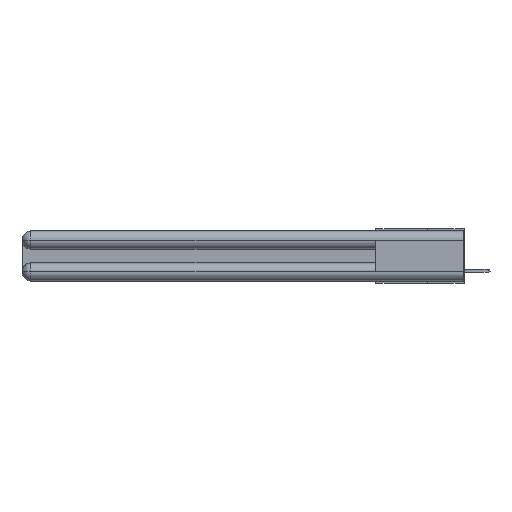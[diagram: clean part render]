
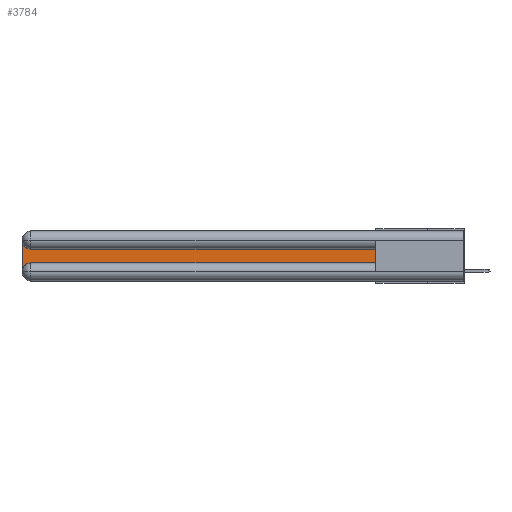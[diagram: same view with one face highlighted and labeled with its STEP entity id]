
A CAD part, left-side view. The second image highlights one B-rep face of the part: STEP entity #3784.
In plain terms, the highlighted planar face has unit normal (-1, 0, 0).
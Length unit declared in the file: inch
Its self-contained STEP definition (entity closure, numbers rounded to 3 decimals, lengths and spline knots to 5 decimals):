
#15 = DIRECTION ( 'NONE',  ( 0., 0., -1. ) ) ;
#426 = VERTEX_POINT ( 'NONE', #9883 ) ;
#629 = ORIENTED_EDGE ( 'NONE', *, *, #4254, .T. ) ;
#3064 = VECTOR ( 'NONE', #15, 39.37008 ) ;
#3088 = DIRECTION ( 'NONE',  ( 0., 0., 1. ) ) ;
#3164 = DIRECTION ( 'NONE',  ( 0., 0., -1. ) ) ;
#3468 = CARTESIAN_POINT ( 'NONE',  ( 0.075, 2.94, -0.2175 ) ) ;
#3784 = ADVANCED_FACE ( 'NONE', ( #25597 ), #5959, .F. ) ;
#4254 = EDGE_CURVE ( 'NONE', #11741, #12722, #5095, .T. ) ;
#5095 = LINE ( 'NONE', #17386, #11734 ) ;
#5959 = PLANE ( 'NONE',  #22119 ) ;
#6924 = CARTESIAN_POINT ( 'NONE',  ( 0.075, 3., -0.2175 ) ) ;
#7071 = CARTESIAN_POINT ( 'NONE',  ( 0.075, 2.94, -0.1225 ) ) ;
#8225 = EDGE_CURVE ( 'NONE', #12722, #13581, #26494, .T. ) ;
#8523 = ORIENTED_EDGE ( 'NONE', *, *, #22843, .T. ) ;
#9883 = CARTESIAN_POINT ( 'NONE',  ( 0.075, 3., -0.0625 ) ) ;
#11553 = DIRECTION ( 'NONE',  ( 0., 1., 0. ) ) ;
#11734 = VECTOR ( 'NONE', #3088, 39.37008 ) ;
#11741 = VERTEX_POINT ( 'NONE', #19174 ) ;
#12194 = VERTEX_POINT ( 'NONE', #16092 ) ;
#12722 = VERTEX_POINT ( 'NONE', #26705 ) ;
#13581 = VERTEX_POINT ( 'NONE', #7071 ) ;
#13681 = CIRCLE ( 'NONE', #25368, 0.06 ) ;
#14512 = CIRCLE ( 'NONE', #22869, 0.06 ) ;
#14736 = CARTESIAN_POINT ( 'NONE',  ( 0.075, 2.94, -0.2775 ) ) ;
#14908 = CARTESIAN_POINT ( 'NONE',  ( 0.075, 2.94, -0.0625 ) ) ;
#15753 = EDGE_CURVE ( 'NONE', #12194, #18931, #14512, .T. ) ;
#16008 = LINE ( 'NONE', #20929, #22916 ) ;
#16092 = CARTESIAN_POINT ( 'NONE',  ( 0.075, 3., -0.2775 ) ) ;
#16308 = VECTOR ( 'NONE', #11553, 39.37008 ) ;
#17386 = CARTESIAN_POINT ( 'NONE',  ( 0.075, 0.6, -0.2175 ) ) ;
#17979 = EDGE_CURVE ( 'NONE', #426, #12194, #29367, .T. ) ;
#18001 = EDGE_LOOP ( 'NONE', ( #21853, #21264, #24338, #20943, #8523, #629 ) ) ;
#18588 = CARTESIAN_POINT ( 'NONE',  ( 0.075, 0.6, -0.1225 ) ) ;
#18931 = VERTEX_POINT ( 'NONE', #3468 ) ;
#19174 = CARTESIAN_POINT ( 'NONE',  ( 0.075, 0.6, -0.2175 ) ) ;
#19418 = DIRECTION ( 'NONE',  ( 1., 0., 0. ) ) ;
#19600 = DIRECTION ( 'NONE',  ( 1., 0., 0. ) ) ;
#20929 = CARTESIAN_POINT ( 'NONE',  ( 0.075, 0.6, -0.2175 ) ) ;
#20943 = ORIENTED_EDGE ( 'NONE', *, *, #15753, .T. ) ;
#21264 = ORIENTED_EDGE ( 'NONE', *, *, #25100, .T. ) ;
#21853 = ORIENTED_EDGE ( 'NONE', *, *, #8225, .T. ) ;
#22119 = AXIS2_PLACEMENT_3D ( 'NONE', #22262, #24613, #26961 ) ;
#22262 = CARTESIAN_POINT ( 'NONE',  ( 0.075, 3., -0.1225 ) ) ;
#22843 = EDGE_CURVE ( 'NONE', #18931, #11741, #16008, .T. ) ;
#22869 = AXIS2_PLACEMENT_3D ( 'NONE', #14736, #19418, #3164 ) ;
#22916 = VECTOR ( 'NONE', #27962, 39.37008 ) ;
#24338 = ORIENTED_EDGE ( 'NONE', *, *, #17979, .T. ) ;
#24613 = DIRECTION ( 'NONE',  ( 1., 0., 0. ) ) ;
#25100 = EDGE_CURVE ( 'NONE', #13581, #426, #13681, .T. ) ;
#25368 = AXIS2_PLACEMENT_3D ( 'NONE', #14908, #19600, #26911 ) ;
#25597 = FACE_OUTER_BOUND ( 'NONE', #18001, .T. ) ;
#26494 = LINE ( 'NONE', #18588, #16308 ) ;
#26705 = CARTESIAN_POINT ( 'NONE',  ( 0.075, 0.6, -0.1225 ) ) ;
#26911 = DIRECTION ( 'NONE',  ( 0., 0., -1. ) ) ;
#26961 = DIRECTION ( 'NONE',  ( 0., 0., -1. ) ) ;
#27962 = DIRECTION ( 'NONE',  ( 0., -1., 0. ) ) ;
#29367 = LINE ( 'NONE', #6924, #3064 ) ;
